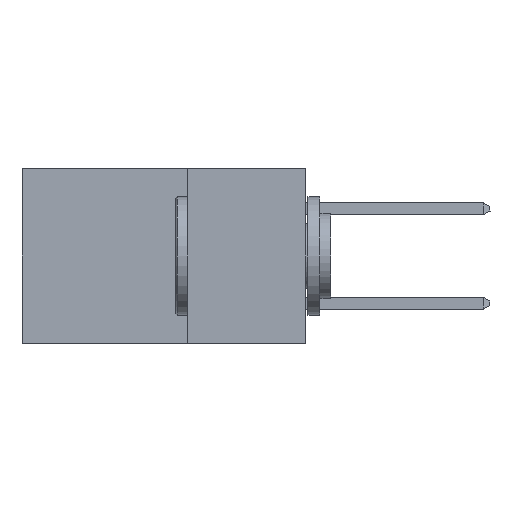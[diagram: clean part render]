
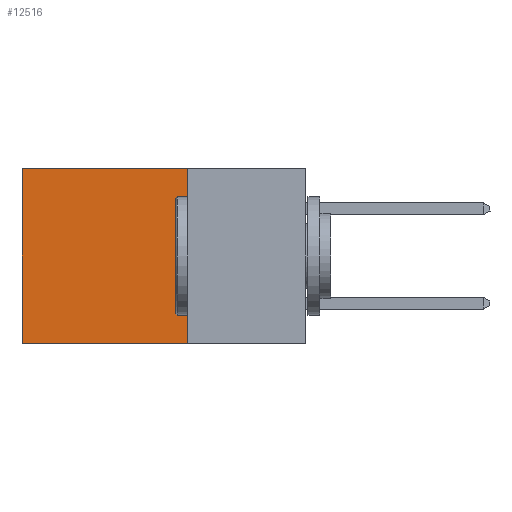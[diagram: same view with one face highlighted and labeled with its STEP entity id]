
A CAD part, left-side view. The second image highlights one B-rep face of the part: STEP entity #12516.
In plain terms, the highlighted planar face has unit normal (-1, 0, 0).
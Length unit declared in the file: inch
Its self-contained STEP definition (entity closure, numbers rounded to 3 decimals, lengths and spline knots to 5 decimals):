
#196 = VECTOR ( 'NONE', #1816, 39.37008 ) ;
#955 = CARTESIAN_POINT ( 'NONE',  ( 0.298, 0.6, 0. ) ) ;
#990 = LINE ( 'NONE', #1453, #4076 ) ;
#1453 = CARTESIAN_POINT ( 'NONE',  ( 0.298, 0.25, 0. ) ) ;
#1477 = EDGE_CURVE ( 'NONE', #6431, #13552, #13729, .T. ) ;
#1480 = CARTESIAN_POINT ( 'NONE',  ( 0.298, 0.6, -0.37 ) ) ;
#1816 = DIRECTION ( 'NONE',  ( 0., 1., 0. ) ) ;
#3537 = LINE ( 'NONE', #10668, #196 ) ;
#4000 = ORIENTED_EDGE ( 'NONE', *, *, #1477, .F. ) ;
#4076 = VECTOR ( 'NONE', #13526, 39.37008 ) ;
#4269 = EDGE_CURVE ( 'NONE', #11211, #6994, #3537, .T. ) ;
#4395 = CARTESIAN_POINT ( 'NONE',  ( 0.298, 0.6, 0. ) ) ;
#5845 = VECTOR ( 'NONE', #7423, 39.37008 ) ;
#6123 = DIRECTION ( 'NONE',  ( 1., 0., 0. ) ) ;
#6178 = AXIS2_PLACEMENT_3D ( 'NONE', #13823, #6123, #13869 ) ;
#6431 = VERTEX_POINT ( 'NONE', #9314 ) ;
#6994 = VERTEX_POINT ( 'NONE', #955 ) ;
#7423 = DIRECTION ( 'NONE',  ( 0., 1., 0. ) ) ;
#7851 = ORIENTED_EDGE ( 'NONE', *, *, #10350, .F. ) ;
#8087 = CARTESIAN_POINT ( 'NONE',  ( 0.298, 0.25, 0. ) ) ;
#8280 = EDGE_LOOP ( 'NONE', ( #9949, #4000, #7851, #9937 ) ) ;
#8286 = PLANE ( 'NONE',  #6178 ) ;
#8489 = CARTESIAN_POINT ( 'NONE',  ( 0.298, 0.25, -0.37 ) ) ;
#8743 = FACE_OUTER_BOUND ( 'NONE', #8280, .T. ) ;
#9037 = LINE ( 'NONE', #4395, #9570 ) ;
#9314 = CARTESIAN_POINT ( 'NONE',  ( 0.298, 0.25, -0.37 ) ) ;
#9570 = VECTOR ( 'NONE', #9845, 39.37008 ) ;
#9845 = DIRECTION ( 'NONE',  ( 0., 0., -1. ) ) ;
#9937 = ORIENTED_EDGE ( 'NONE', *, *, #4269, .T. ) ;
#9949 = ORIENTED_EDGE ( 'NONE', *, *, #14402, .T. ) ;
#10350 = EDGE_CURVE ( 'NONE', #11211, #6431, #990, .T. ) ;
#10668 = CARTESIAN_POINT ( 'NONE',  ( 0.298, 0.25, 0. ) ) ;
#11211 = VERTEX_POINT ( 'NONE', #8087 ) ;
#12516 = ADVANCED_FACE ( 'NONE', ( #8743 ), #8286, .F. ) ;
#13526 = DIRECTION ( 'NONE',  ( 0., 0., -1. ) ) ;
#13552 = VERTEX_POINT ( 'NONE', #1480 ) ;
#13729 = LINE ( 'NONE', #8489, #5845 ) ;
#13823 = CARTESIAN_POINT ( 'NONE',  ( 0.298, 0.25, 0. ) ) ;
#13869 = DIRECTION ( 'NONE',  ( 0., 0., -1. ) ) ;
#14402 = EDGE_CURVE ( 'NONE', #6994, #13552, #9037, .T. ) ;
